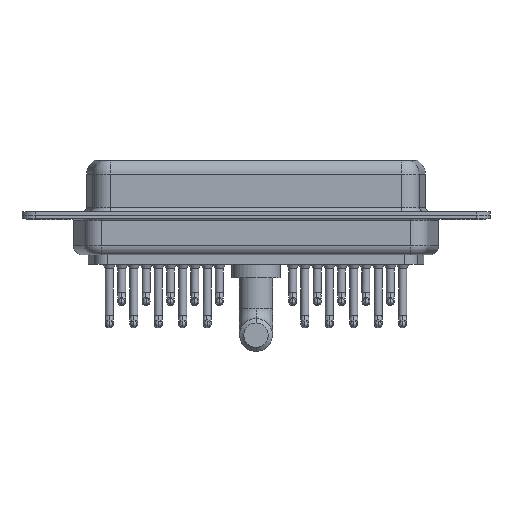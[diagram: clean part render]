
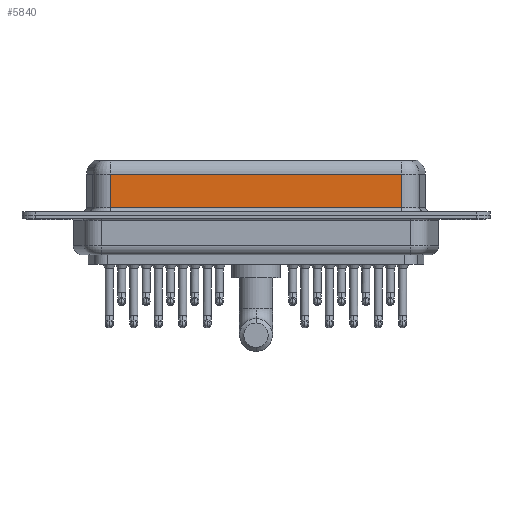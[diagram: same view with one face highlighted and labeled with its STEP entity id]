
A CAD part, front view. The second image highlights one B-rep face of the part: STEP entity #5840.
In plain terms, the highlighted planar face has unit normal (0, -1, 0).
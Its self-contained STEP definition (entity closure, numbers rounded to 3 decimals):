
#34 = VECTOR ( 'NONE', #10636, 1000. ) ;
#156 = ORIENTED_EDGE ( 'NONE', *, *, #3468, .F. ) ;
#882 = CARTESIAN_POINT ( 'NONE',  ( 40.037, -3.95, 4.65 ) ) ;
#1813 = CARTESIAN_POINT ( 'NONE',  ( 7.013, -3.95, 0.9 ) ) ;
#1858 = VERTEX_POINT ( 'NONE', #1813 ) ;
#1912 = VECTOR ( 'NONE', #8772, 1000. ) ;
#2627 = ORIENTED_EDGE ( 'NONE', *, *, #5706, .T. ) ;
#2782 = CARTESIAN_POINT ( 'NONE',  ( 40.037, -3.95, 0.9 ) ) ;
#3468 = EDGE_CURVE ( 'NONE', #8423, #6543, #13439, .T. ) ;
#4796 = DIRECTION ( 'NONE',  ( 0., 0., 1. ) ) ;
#5706 = EDGE_CURVE ( 'NONE', #1858, #6543, #7743, .T. ) ;
#5840 = ADVANCED_FACE ( 'NONE', ( #13260 ), #17794, .F. ) ;
#6543 = VERTEX_POINT ( 'NONE', #8561 ) ;
#7681 = VECTOR ( 'NONE', #9346, 1000. ) ;
#7743 = LINE ( 'NONE', #2782, #7681 ) ;
#7898 = EDGE_CURVE ( 'NONE', #8423, #14231, #10425, .T. ) ;
#8379 = DIRECTION ( 'NONE',  ( 0., 1., 0. ) ) ;
#8423 = VERTEX_POINT ( 'NONE', #882 ) ;
#8561 = CARTESIAN_POINT ( 'NONE',  ( 40.037, -3.95, 0.9 ) ) ;
#8772 = DIRECTION ( 'NONE',  ( 0., 0., -1. ) ) ;
#8843 = DIRECTION ( 'NONE',  ( -1., 0., 0. ) ) ;
#9346 = DIRECTION ( 'NONE',  ( 1., 0., 0. ) ) ;
#9956 = EDGE_LOOP ( 'NONE', ( #156, #12765, #16059, #2627 ) ) ;
#10067 = AXIS2_PLACEMENT_3D ( 'NONE', #19465, #8379, #4796 ) ;
#10266 = CARTESIAN_POINT ( 'NONE',  ( 40.037, -3.95, 6.4 ) ) ;
#10425 = LINE ( 'NONE', #19614, #14337 ) ;
#10636 = DIRECTION ( 'NONE',  ( 0., 0., -1. ) ) ;
#12016 = LINE ( 'NONE', #15407, #34 ) ;
#12765 = ORIENTED_EDGE ( 'NONE', *, *, #7898, .T. ) ;
#13260 = FACE_OUTER_BOUND ( 'NONE', #9956, .T. ) ;
#13439 = LINE ( 'NONE', #10266, #1912 ) ;
#14231 = VERTEX_POINT ( 'NONE', #18669 ) ;
#14337 = VECTOR ( 'NONE', #8843, 1000. ) ;
#15407 = CARTESIAN_POINT ( 'NONE',  ( 7.013, -3.95, 6.4 ) ) ;
#16059 = ORIENTED_EDGE ( 'NONE', *, *, #17732, .T. ) ;
#17732 = EDGE_CURVE ( 'NONE', #14231, #1858, #12016, .T. ) ;
#17794 = PLANE ( 'NONE',  #10067 ) ;
#18669 = CARTESIAN_POINT ( 'NONE',  ( 7.013, -3.95, 4.65 ) ) ;
#19465 = CARTESIAN_POINT ( 'NONE',  ( 40.037, -3.95, 6.4 ) ) ;
#19614 = CARTESIAN_POINT ( 'NONE',  ( 40.037, -3.95, 4.65 ) ) ;
